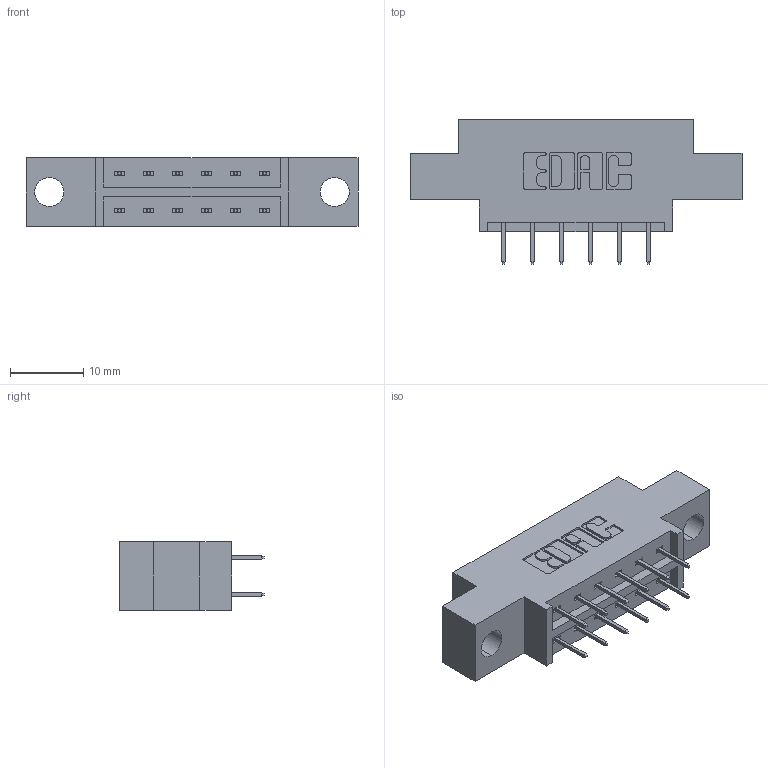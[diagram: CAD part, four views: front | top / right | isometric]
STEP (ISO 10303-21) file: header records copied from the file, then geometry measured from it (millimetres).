
FILE_DESCRIPTION (( 'STEP AP203' ), '1' );
FILE_NAME ('333-012-524-804.STEP', '2018-08-01T00:15:19', ( '' ), ( '' ), 'SwSTEP 2.0', 'SolidWorks 2016', '' );
FILE_SCHEMA (( 'CONFIG_CONTROL_DESIGN' ));
Length unit declared in the file: inch
Products named in the file (3): 333 Part_Offset - .156 Dia - TH; 345-292-001_345-293-124; 333-012-524-804
Assembly tree (13 placements, depth 2):
  333-012-524-804
    333 Part_Offset - .156 Dia - TH
    345-292-001_345-293-124  x12
Bounding box: 45.31 x 19.69 x 9.4 mm (x, y, z)
Volume: 3955.8 mm3; surface area: 4255.6 mm2
Topology: 13 solids, 13 shells, 790 faces, 2231 edges, 1438 vertices
Faces by surface type: plane 578, cylinder 212
Entity records: 8725 total; most frequent: CARTESIAN_POINT 1490, ORIENTED_EDGE 1426, DIRECTION 1337, EDGE_CURVE 713, LINE 589, VECTOR 589, VERTEX_POINT 470, AXIS2_PLACEMENT_3D 374
